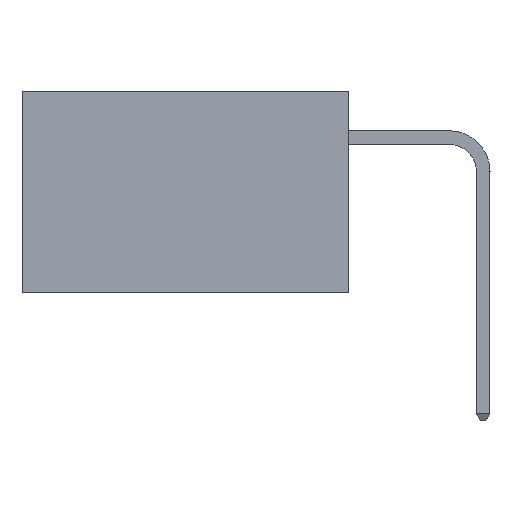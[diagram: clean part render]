
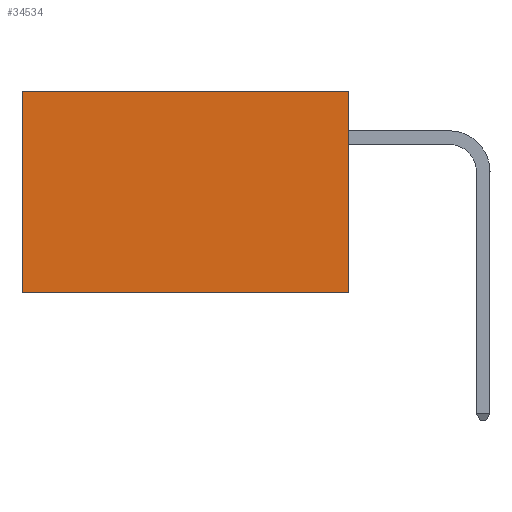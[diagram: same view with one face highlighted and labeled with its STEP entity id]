
A CAD part, left-side view. The second image highlights one B-rep face of the part: STEP entity #34534.
In plain terms, the highlighted planar face has unit normal (-1, 0, 0).
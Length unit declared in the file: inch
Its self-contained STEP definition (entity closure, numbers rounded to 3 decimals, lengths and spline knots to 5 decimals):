
#661 = VERTEX_POINT ( 'NONE', #26114 ) ;
#1309 = DIRECTION ( 'NONE',  ( 0., 0., -1. ) ) ;
#2537 = VECTOR ( 'NONE', #9211, 39.37008 ) ;
#3852 = CARTESIAN_POINT ( 'NONE',  ( 0.2875, 0., -0.37 ) ) ;
#4258 = DIRECTION ( 'NONE',  ( 0., 1., 0. ) ) ;
#5892 = AXIS2_PLACEMENT_3D ( 'NONE', #11599, #34710, #14946 ) ;
#7315 = FACE_OUTER_BOUND ( 'NONE', #21109, .T. ) ;
#9211 = DIRECTION ( 'NONE',  ( 0., 0., -1. ) ) ;
#10998 = CARTESIAN_POINT ( 'NONE',  ( 0.2875, 0.6, -0.37 ) ) ;
#11568 = LINE ( 'NONE', #29027, #2537 ) ;
#11599 = CARTESIAN_POINT ( 'NONE',  ( 0.2875, 0., 0. ) ) ;
#11664 = EDGE_CURVE ( 'NONE', #26368, #36948, #11568, .T. ) ;
#13085 = VECTOR ( 'NONE', #1309, 39.37008 ) ;
#14679 = DIRECTION ( 'NONE',  ( 0., 1., 0. ) ) ;
#14946 = DIRECTION ( 'NONE',  ( 0., 0., -1. ) ) ;
#15154 = LINE ( 'NONE', #27915, #13085 ) ;
#17147 = CARTESIAN_POINT ( 'NONE',  ( 0.2875, 0., 0. ) ) ;
#18269 = VERTEX_POINT ( 'NONE', #10998 ) ;
#18281 = VECTOR ( 'NONE', #4258, 39.37008 ) ;
#19992 = ORIENTED_EDGE ( 'NONE', *, *, #33922, .F. ) ;
#21109 = EDGE_LOOP ( 'NONE', ( #28064, #19992, #30156, #22936 ) ) ;
#22936 = ORIENTED_EDGE ( 'NONE', *, *, #24985, .T. ) ;
#23510 = VECTOR ( 'NONE', #14679, 39.37008 ) ;
#24523 = CARTESIAN_POINT ( 'NONE',  ( 0.2875, 0., -0.37 ) ) ;
#24985 = EDGE_CURVE ( 'NONE', #26368, #661, #36840, .T. ) ;
#26114 = CARTESIAN_POINT ( 'NONE',  ( 0.2875, 0.6, 0. ) ) ;
#26368 = VERTEX_POINT ( 'NONE', #17147 ) ;
#26555 = EDGE_CURVE ( 'NONE', #661, #18269, #15154, .T. ) ;
#27915 = CARTESIAN_POINT ( 'NONE',  ( 0.2875, 0.6, 0. ) ) ;
#28064 = ORIENTED_EDGE ( 'NONE', *, *, #26555, .T. ) ;
#29027 = CARTESIAN_POINT ( 'NONE',  ( 0.2875, 0., 0. ) ) ;
#30156 = ORIENTED_EDGE ( 'NONE', *, *, #11664, .F. ) ;
#31427 = PLANE ( 'NONE',  #5892 ) ;
#33922 = EDGE_CURVE ( 'NONE', #36948, #18269, #42070, .T. ) ;
#34534 = ADVANCED_FACE ( 'NONE', ( #7315 ), #31427, .F. ) ;
#34710 = DIRECTION ( 'NONE',  ( 1., 0., 0. ) ) ;
#36840 = LINE ( 'NONE', #37419, #18281 ) ;
#36948 = VERTEX_POINT ( 'NONE', #3852 ) ;
#37419 = CARTESIAN_POINT ( 'NONE',  ( 0.2875, 0., 0. ) ) ;
#42070 = LINE ( 'NONE', #24523, #23510 ) ;
